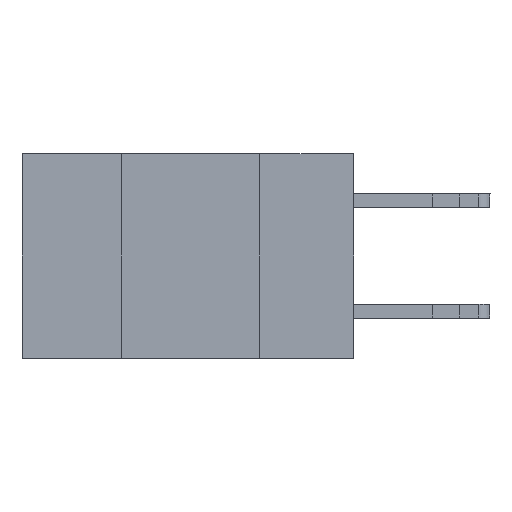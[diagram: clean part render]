
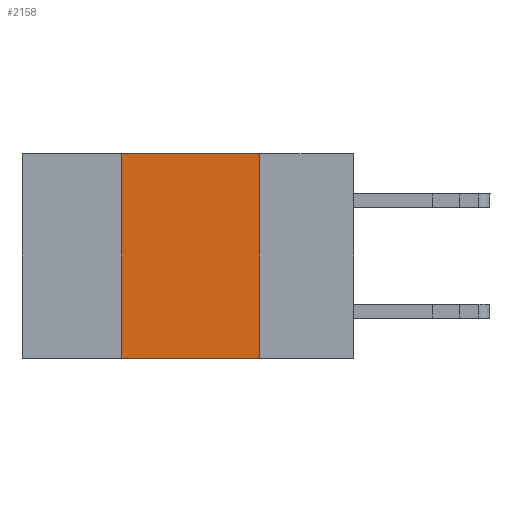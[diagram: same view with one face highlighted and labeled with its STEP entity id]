
A CAD part, left-side view. The second image highlights one B-rep face of the part: STEP entity #2158.
In plain terms, the highlighted planar face has unit normal (-1, 0, 0).
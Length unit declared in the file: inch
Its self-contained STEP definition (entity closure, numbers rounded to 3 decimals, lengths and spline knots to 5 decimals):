
#909 = CARTESIAN_POINT ( 'NONE',  ( 0., 0.17, 0. ) ) ;
#2158 = ADVANCED_FACE ( 'NONE', ( #16402 ), #17301, .F. ) ;
#2276 = EDGE_CURVE ( 'NONE', #17492, #22199, #9437, .T. ) ;
#4053 = EDGE_CURVE ( 'NONE', #16634, #22199, #11759, .T. ) ;
#5093 = VERTEX_POINT ( 'NONE', #5828 ) ;
#5243 = CARTESIAN_POINT ( 'NONE',  ( 0., 0.6, -0.37 ) ) ;
#5828 = CARTESIAN_POINT ( 'NONE',  ( 0., 0.42, 0. ) ) ;
#6198 = CARTESIAN_POINT ( 'NONE',  ( 0., 0.6, 0. ) ) ;
#6845 = AXIS2_PLACEMENT_3D ( 'NONE', #19249, #21208, #23179 ) ;
#7200 = DIRECTION ( 'NONE',  ( 0., -1., 0. ) ) ;
#7334 = VECTOR ( 'NONE', #23869, 39.37008 ) ;
#9437 = LINE ( 'NONE', #17522, #18843 ) ;
#10131 = DIRECTION ( 'NONE',  ( 0., -1., 0. ) ) ;
#10615 = ORIENTED_EDGE ( 'NONE', *, *, #2276, .F. ) ;
#11301 = ORIENTED_EDGE ( 'NONE', *, *, #4053, .T. ) ;
#11392 = EDGE_CURVE ( 'NONE', #16634, #5093, #22235, .T. ) ;
#11759 = LINE ( 'NONE', #5243, #15975 ) ;
#12308 = EDGE_CURVE ( 'NONE', #5093, #17492, #18849, .T. ) ;
#13479 = ORIENTED_EDGE ( 'NONE', *, *, #12308, .F. ) ;
#13545 = EDGE_LOOP ( 'NONE', ( #10615, #13479, #25119, #11301 ) ) ;
#15975 = VECTOR ( 'NONE', #7200, 39.37008 ) ;
#16402 = FACE_OUTER_BOUND ( 'NONE', #13545, .T. ) ;
#16634 = VERTEX_POINT ( 'NONE', #19571 ) ;
#17301 = PLANE ( 'NONE',  #6845 ) ;
#17492 = VERTEX_POINT ( 'NONE', #909 ) ;
#17522 = CARTESIAN_POINT ( 'NONE',  ( 0., 0.17, 0. ) ) ;
#18198 = CARTESIAN_POINT ( 'NONE',  ( 0., 0.17, -0.37 ) ) ;
#18218 = VECTOR ( 'NONE', #10131, 39.37008 ) ;
#18843 = VECTOR ( 'NONE', #23480, 39.37008 ) ;
#18849 = LINE ( 'NONE', #6198, #18218 ) ;
#19249 = CARTESIAN_POINT ( 'NONE',  ( 0., 0.6, 0. ) ) ;
#19571 = CARTESIAN_POINT ( 'NONE',  ( 0., 0.42, -0.37 ) ) ;
#21208 = DIRECTION ( 'NONE',  ( 1., 0., 0. ) ) ;
#22199 = VERTEX_POINT ( 'NONE', #18198 ) ;
#22235 = LINE ( 'NONE', #23716, #7334 ) ;
#23179 = DIRECTION ( 'NONE',  ( 0., 0., -1. ) ) ;
#23480 = DIRECTION ( 'NONE',  ( 0., 0., -1. ) ) ;
#23716 = CARTESIAN_POINT ( 'NONE',  ( 0., 0.42, 0. ) ) ;
#23869 = DIRECTION ( 'NONE',  ( 0., 0., 1. ) ) ;
#25119 = ORIENTED_EDGE ( 'NONE', *, *, #11392, .F. ) ;
